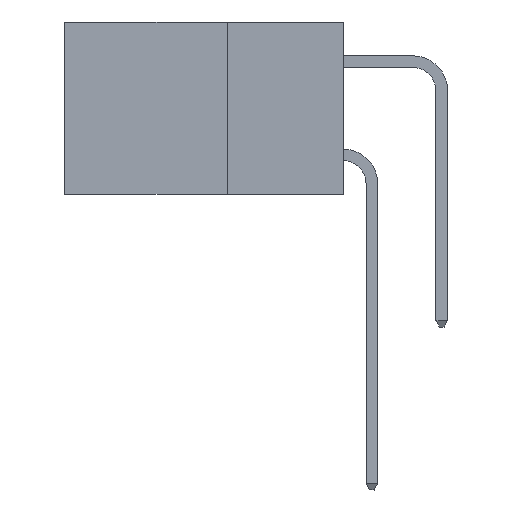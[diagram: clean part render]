
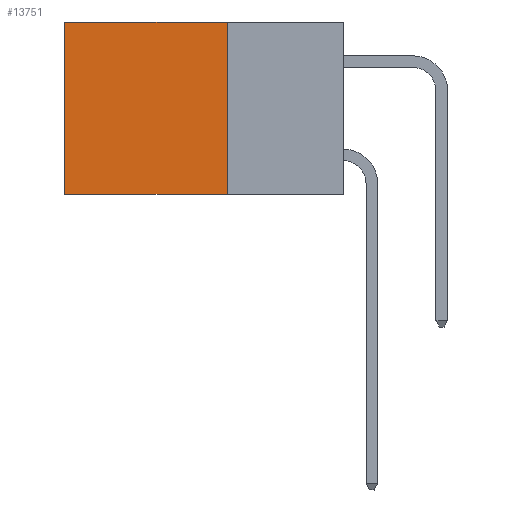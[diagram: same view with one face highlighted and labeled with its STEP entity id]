
A CAD part, left-side view. The second image highlights one B-rep face of the part: STEP entity #13751.
In plain terms, the highlighted planar face has unit normal (-1, 0, 0).
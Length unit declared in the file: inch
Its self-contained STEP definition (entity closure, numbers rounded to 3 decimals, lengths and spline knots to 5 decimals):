
#258 = FACE_OUTER_BOUND ( 'NONE', #12820, .T. ) ;
#570 = LINE ( 'NONE', #673, #13004 ) ;
#673 = CARTESIAN_POINT ( 'NONE',  ( 0.298, 0.25, 0. ) ) ;
#728 = DIRECTION ( 'NONE',  ( 0., 1., 0. ) ) ;
#982 = CARTESIAN_POINT ( 'NONE',  ( 0.298, 0.6, 0. ) ) ;
#1807 = DIRECTION ( 'NONE',  ( 0., 0., -1. ) ) ;
#2084 = ORIENTED_EDGE ( 'NONE', *, *, #5199, .F. ) ;
#2223 = EDGE_CURVE ( 'NONE', #14204, #14423, #12429, .T. ) ;
#4401 = CARTESIAN_POINT ( 'NONE',  ( 0.298, 0.25, 0. ) ) ;
#4672 = DIRECTION ( 'NONE',  ( 0., 0., -1. ) ) ;
#4900 = ORIENTED_EDGE ( 'NONE', *, *, #7055, .T. ) ;
#5120 = ORIENTED_EDGE ( 'NONE', *, *, #2223, .T. ) ;
#5159 = CARTESIAN_POINT ( 'NONE',  ( 0.298, 0.25, 0. ) ) ;
#5178 = LINE ( 'NONE', #6693, #11186 ) ;
#5199 = EDGE_CURVE ( 'NONE', #8435, #14423, #5178, .T. ) ;
#5727 = EDGE_CURVE ( 'NONE', #8800, #8435, #10096, .T. ) ;
#6572 = CARTESIAN_POINT ( 'NONE',  ( 0.298, 0.25, 0. ) ) ;
#6693 = CARTESIAN_POINT ( 'NONE',  ( 0.298, 0.25, -0.37 ) ) ;
#6791 = VECTOR ( 'NONE', #4672, 39.37008 ) ;
#6947 = CARTESIAN_POINT ( 'NONE',  ( 0.298, 0.25, -0.37 ) ) ;
#7055 = EDGE_CURVE ( 'NONE', #8800, #14204, #570, .T. ) ;
#7832 = PLANE ( 'NONE',  #12233 ) ;
#8435 = VERTEX_POINT ( 'NONE', #6947 ) ;
#8745 = CARTESIAN_POINT ( 'NONE',  ( 0.298, 0.6, 0. ) ) ;
#8800 = VERTEX_POINT ( 'NONE', #5159 ) ;
#9080 = DIRECTION ( 'NONE',  ( 1., 0., 0. ) ) ;
#9187 = DIRECTION ( 'NONE',  ( 0., 1., 0. ) ) ;
#10096 = LINE ( 'NONE', #4401, #13578 ) ;
#11186 = VECTOR ( 'NONE', #9187, 39.37008 ) ;
#11578 = DIRECTION ( 'NONE',  ( 0., 0., -1. ) ) ;
#12233 = AXIS2_PLACEMENT_3D ( 'NONE', #6572, #9080, #1807 ) ;
#12429 = LINE ( 'NONE', #982, #6791 ) ;
#12820 = EDGE_LOOP ( 'NONE', ( #5120, #2084, #15111, #4900 ) ) ;
#13004 = VECTOR ( 'NONE', #728, 39.37008 ) ;
#13578 = VECTOR ( 'NONE', #11578, 39.37008 ) ;
#13751 = ADVANCED_FACE ( 'NONE', ( #258 ), #7832, .F. ) ;
#13846 = CARTESIAN_POINT ( 'NONE',  ( 0.298, 0.6, -0.37 ) ) ;
#14204 = VERTEX_POINT ( 'NONE', #8745 ) ;
#14423 = VERTEX_POINT ( 'NONE', #13846 ) ;
#15111 = ORIENTED_EDGE ( 'NONE', *, *, #5727, .F. ) ;
